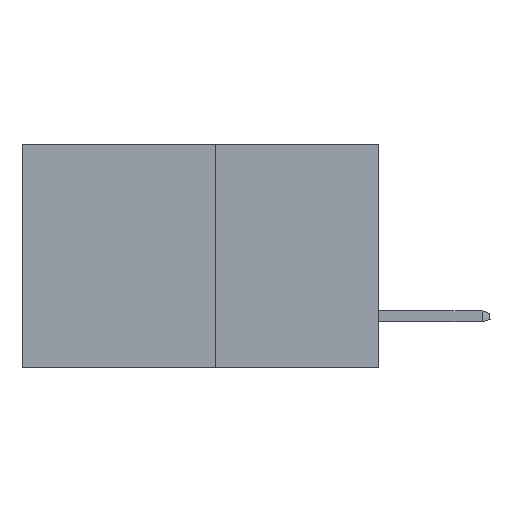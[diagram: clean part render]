
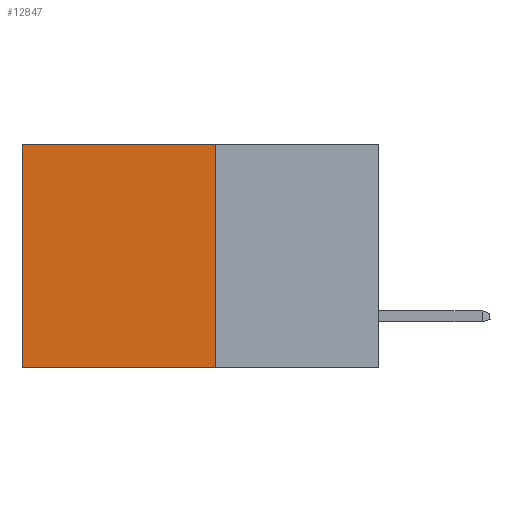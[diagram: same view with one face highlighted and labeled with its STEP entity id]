
A CAD part, left-side view. The second image highlights one B-rep face of the part: STEP entity #12847.
In plain terms, the highlighted planar face has unit normal (-1, 0, 0).
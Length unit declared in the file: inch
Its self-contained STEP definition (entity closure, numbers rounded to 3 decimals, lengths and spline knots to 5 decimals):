
#165 = VERTEX_POINT ( 'NONE', #23958 ) ;
#725 = LINE ( 'NONE', #22278, #22358 ) ;
#1711 = ORIENTED_EDGE ( 'NONE', *, *, #18703, .F. ) ;
#2471 = AXIS2_PLACEMENT_3D ( 'NONE', #11447, #9638, #9546 ) ;
#3816 = VECTOR ( 'NONE', #13108, 39.37008 ) ;
#4694 = ORIENTED_EDGE ( 'NONE', *, *, #15458, .T. ) ;
#4902 = ORIENTED_EDGE ( 'NONE', *, *, #11148, .F. ) ;
#5223 = DIRECTION ( 'NONE',  ( 0., 1., 0. ) ) ;
#6061 = DIRECTION ( 'NONE',  ( 0., 1., 0. ) ) ;
#6189 = VECTOR ( 'NONE', #13648, 39.37008 ) ;
#8110 = LINE ( 'NONE', #11481, #6189 ) ;
#8782 = VECTOR ( 'NONE', #5223, 39.37008 ) ;
#9546 = DIRECTION ( 'NONE',  ( 0., 0., -1. ) ) ;
#9638 = DIRECTION ( 'NONE',  ( 1., 0., 0. ) ) ;
#10066 = PLANE ( 'NONE',  #2471 ) ;
#11148 = EDGE_CURVE ( 'NONE', #165, #11243, #20082, .T. ) ;
#11243 = VERTEX_POINT ( 'NONE', #12135 ) ;
#11447 = CARTESIAN_POINT ( 'NONE',  ( 0.277, 0.27, -0.37 ) ) ;
#11481 = CARTESIAN_POINT ( 'NONE',  ( 0.277, 0.59, -0.37 ) ) ;
#12135 = CARTESIAN_POINT ( 'NONE',  ( 0.277, 0.27, -0.37 ) ) ;
#12847 = ADVANCED_FACE ( 'NONE', ( #18730 ), #10066, .F. ) ;
#13108 = DIRECTION ( 'NONE',  ( 0., 0., -1. ) ) ;
#13204 = CARTESIAN_POINT ( 'NONE',  ( 0.277, 0.27, -0.37 ) ) ;
#13465 = VERTEX_POINT ( 'NONE', #25313 ) ;
#13648 = DIRECTION ( 'NONE',  ( 0., 0., -1. ) ) ;
#14942 = EDGE_LOOP ( 'NONE', ( #26224, #1711, #4902, #4694 ) ) ;
#15458 = EDGE_CURVE ( 'NONE', #165, #25155, #24248, .T. ) ;
#17445 = CARTESIAN_POINT ( 'NONE',  ( 0.277, 0.27, 0. ) ) ;
#18703 = EDGE_CURVE ( 'NONE', #11243, #13465, #725, .T. ) ;
#18730 = FACE_OUTER_BOUND ( 'NONE', #14942, .T. ) ;
#19119 = CARTESIAN_POINT ( 'NONE',  ( 0.277, 0.59, 0. ) ) ;
#20082 = LINE ( 'NONE', #13204, #3816 ) ;
#21796 = EDGE_CURVE ( 'NONE', #25155, #13465, #8110, .T. ) ;
#22278 = CARTESIAN_POINT ( 'NONE',  ( 0.277, 0.27, -0.37 ) ) ;
#22358 = VECTOR ( 'NONE', #6061, 39.37008 ) ;
#23958 = CARTESIAN_POINT ( 'NONE',  ( 0.277, 0.27, 0. ) ) ;
#24248 = LINE ( 'NONE', #17445, #8782 ) ;
#25155 = VERTEX_POINT ( 'NONE', #19119 ) ;
#25313 = CARTESIAN_POINT ( 'NONE',  ( 0.277, 0.59, -0.37 ) ) ;
#26224 = ORIENTED_EDGE ( 'NONE', *, *, #21796, .T. ) ;
